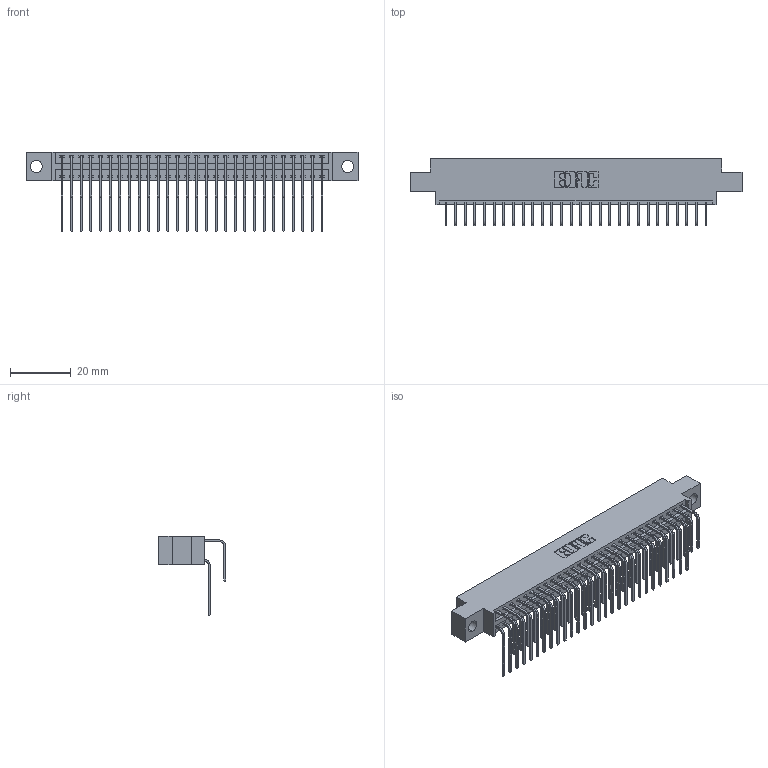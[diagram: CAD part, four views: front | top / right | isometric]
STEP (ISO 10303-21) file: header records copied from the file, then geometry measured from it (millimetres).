
FILE_DESCRIPTION (( 'STEP AP203' ), '1' );
FILE_NAME ('346-056-558-804.STEP', '2022-05-21T06:46:02', ( '' ), ( '' ), 'SwSTEP 2.0', 'SolidWorks 2020', '' );
FILE_SCHEMA (( 'CONFIG_CONTROL_DESIGN' ));
Length unit declared in the file: inch
Products named in the file (4): 346-056-558-804; 346 Part_0.170 Offset - 0.156 Dia-TH; 345-292-001_558 Tail - 2; 345-292-001_558 559 Tail - 1
Assembly tree (57 placements, depth 2):
  346-056-558-804
    346 Part_0.170 Offset - 0.156 Dia-TH
    345-292-001_558 559 Tail - 1  x28
    345-292-001_558 Tail - 2  x28
Bounding box: 109.47 x 22.16 x 26.16 mm (x, y, z)
Volume: 10628.8 mm3; surface area: 15967.3 mm2
Topology: 57 solids, 57 shells, 3164 faces, 9393 edges, 6186 vertices
Faces by surface type: plane 2166, cylinder 998
Entity records: 22493 total; most frequent: CARTESIAN_POINT 3785, ORIENTED_EDGE 3666, DIRECTION 3357, EDGE_CURVE 1833, VECTOR 1549, LINE 1549, VERTEX_POINT 1218, AXIS2_PLACEMENT_3D 904
